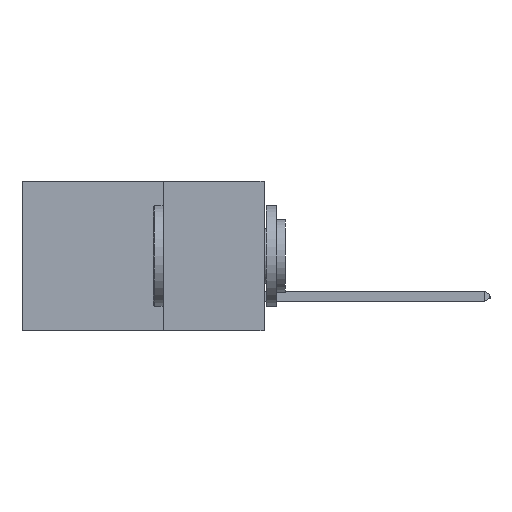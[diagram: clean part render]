
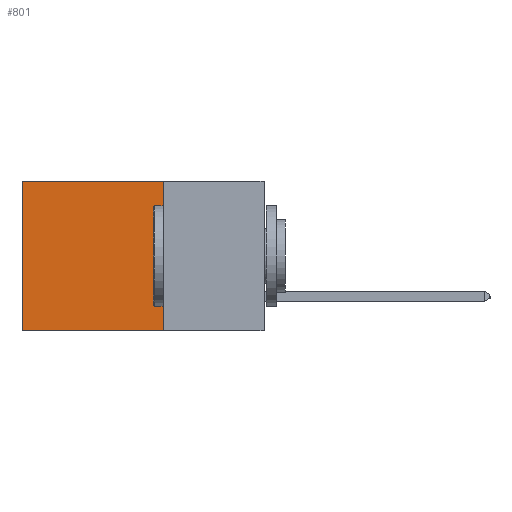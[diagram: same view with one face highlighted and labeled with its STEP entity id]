
A CAD part, left-side view. The second image highlights one B-rep face of the part: STEP entity #801.
In plain terms, the highlighted planar face has unit normal (-1, 0, 0).
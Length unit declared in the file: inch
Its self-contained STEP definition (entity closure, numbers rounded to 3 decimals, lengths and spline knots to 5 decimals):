
#728 = CARTESIAN_POINT ( 'NONE',  ( 0.298, 0.25, 0. ) ) ;
#801 = ADVANCED_FACE ( 'NONE', ( #7081 ), #10492, .F. ) ;
#1017 = VERTEX_POINT ( 'NONE', #7452 ) ;
#1404 = VECTOR ( 'NONE', #9982, 39.37008 ) ;
#1898 = LINE ( 'NONE', #7170, #7075 ) ;
#2202 = CARTESIAN_POINT ( 'NONE',  ( 0.298, 0.25, 0. ) ) ;
#2386 = EDGE_CURVE ( 'NONE', #1017, #3505, #9035, .T. ) ;
#2789 = EDGE_LOOP ( 'NONE', ( #3966, #3561, #5713, #5889 ) ) ;
#3448 = CARTESIAN_POINT ( 'NONE',  ( 0.298, 0.6, -0.37 ) ) ;
#3505 = VERTEX_POINT ( 'NONE', #3448 ) ;
#3561 = ORIENTED_EDGE ( 'NONE', *, *, #9855, .F. ) ;
#3577 = CARTESIAN_POINT ( 'NONE',  ( 0.298, 0.25, 0. ) ) ;
#3966 = ORIENTED_EDGE ( 'NONE', *, *, #2386, .T. ) ;
#4666 = LINE ( 'NONE', #728, #11751 ) ;
#4753 = DIRECTION ( 'NONE',  ( 1., 0., 0. ) ) ;
#5713 = ORIENTED_EDGE ( 'NONE', *, *, #7594, .F. ) ;
#5889 = ORIENTED_EDGE ( 'NONE', *, *, #8846, .T. ) ;
#6032 = DIRECTION ( 'NONE',  ( 0., 0., -1. ) ) ;
#6608 = DIRECTION ( 'NONE',  ( 0., 1., 0. ) ) ;
#6817 = VECTOR ( 'NONE', #9771, 39.37008 ) ;
#7075 = VECTOR ( 'NONE', #11652, 39.37008 ) ;
#7081 = FACE_OUTER_BOUND ( 'NONE', #2789, .T. ) ;
#7153 = AXIS2_PLACEMENT_3D ( 'NONE', #3577, #4753, #6032 ) ;
#7170 = CARTESIAN_POINT ( 'NONE',  ( 0.298, 0.25, -0.37 ) ) ;
#7452 = CARTESIAN_POINT ( 'NONE',  ( 0.298, 0.6, 0. ) ) ;
#7594 = EDGE_CURVE ( 'NONE', #7659, #7996, #11899, .T. ) ;
#7659 = VERTEX_POINT ( 'NONE', #8948 ) ;
#7996 = VERTEX_POINT ( 'NONE', #11195 ) ;
#8846 = EDGE_CURVE ( 'NONE', #7659, #1017, #4666, .T. ) ;
#8948 = CARTESIAN_POINT ( 'NONE',  ( 0.298, 0.25, 0. ) ) ;
#9035 = LINE ( 'NONE', #9373, #1404 ) ;
#9373 = CARTESIAN_POINT ( 'NONE',  ( 0.298, 0.6, 0. ) ) ;
#9771 = DIRECTION ( 'NONE',  ( 0., 0., -1. ) ) ;
#9855 = EDGE_CURVE ( 'NONE', #7996, #3505, #1898, .T. ) ;
#9982 = DIRECTION ( 'NONE',  ( 0., 0., -1. ) ) ;
#10492 = PLANE ( 'NONE',  #7153 ) ;
#11195 = CARTESIAN_POINT ( 'NONE',  ( 0.298, 0.25, -0.37 ) ) ;
#11652 = DIRECTION ( 'NONE',  ( 0., 1., 0. ) ) ;
#11751 = VECTOR ( 'NONE', #6608, 39.37008 ) ;
#11899 = LINE ( 'NONE', #2202, #6817 ) ;
